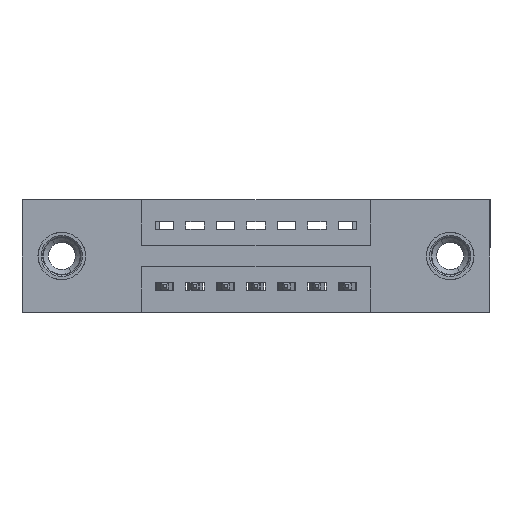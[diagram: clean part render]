
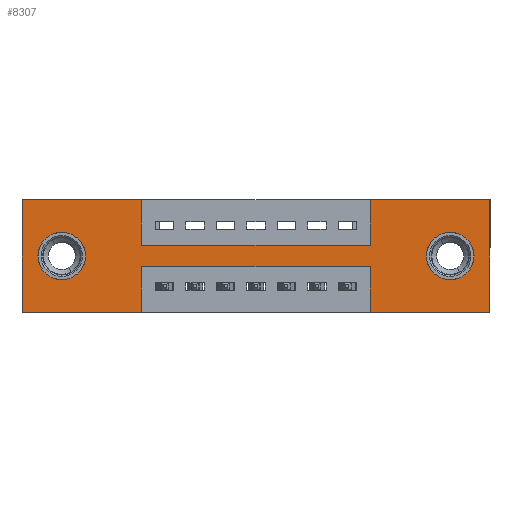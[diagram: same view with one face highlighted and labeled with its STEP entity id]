
A CAD part, front view. The second image highlights one B-rep face of the part: STEP entity #8307.
In plain terms, the highlighted planar face has unit normal (0, -1, 0).
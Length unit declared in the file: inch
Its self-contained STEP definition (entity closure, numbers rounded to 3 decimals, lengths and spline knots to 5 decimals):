
#32 = VERTEX_POINT ( 'NONE', #416 ) ;
#128 = ORIENTED_EDGE ( 'NONE', *, *, #7319, .F. ) ;
#147 = DIRECTION ( 'NONE',  ( 0., 0., -1. ) ) ;
#178 = ORIENTED_EDGE ( 'NONE', *, *, #6725, .F. ) ;
#416 = CARTESIAN_POINT ( 'NONE',  ( 1.1425, 0., -0.37 ) ) ;
#437 = VERTEX_POINT ( 'NONE', #9401 ) ;
#491 = DIRECTION ( 'NONE',  ( 0., -1., 0. ) ) ;
#537 = CARTESIAN_POINT ( 'NONE',  ( 1.535, 0., 0. ) ) ;
#649 = PLANE ( 'NONE',  #10290 ) ;
#993 = CARTESIAN_POINT ( 'NONE',  ( 1.535, 0., 0. ) ) ;
#1049 = EDGE_CURVE ( 'NONE', #6370, #8377, #3163, .T. ) ;
#1101 = DIRECTION ( 'NONE',  ( 0., 0., -1. ) ) ;
#1355 = DIRECTION ( 'NONE',  ( -1., 0., 0. ) ) ;
#1365 = DIRECTION ( 'NONE',  ( 0., 0., -1. ) ) ;
#1394 = CARTESIAN_POINT ( 'NONE',  ( 0.3925, 0., -0.15 ) ) ;
#1626 = CARTESIAN_POINT ( 'NONE',  ( 1.1425, 0., 0. ) ) ;
#1675 = EDGE_CURVE ( 'NONE', #11949, #1896, #2413, .T. ) ;
#1891 = LINE ( 'NONE', #5051, #7633 ) ;
#1896 = VERTEX_POINT ( 'NONE', #8954 ) ;
#1905 = CARTESIAN_POINT ( 'NONE',  ( 0.3925, 0., -0.22 ) ) ;
#1907 = LINE ( 'NONE', #11423, #2347 ) ;
#2055 = VECTOR ( 'NONE', #5692, 39.37008 ) ;
#2180 = VERTEX_POINT ( 'NONE', #1626 ) ;
#2265 = DIRECTION ( 'NONE',  ( 0., 0., 1. ) ) ;
#2316 = CARTESIAN_POINT ( 'NONE',  ( 0.3925, 0., -0.37 ) ) ;
#2347 = VECTOR ( 'NONE', #7662, 39.37008 ) ;
#2413 = LINE ( 'NONE', #993, #10087 ) ;
#2418 = CARTESIAN_POINT ( 'NONE',  ( 0., 0., -0.37 ) ) ;
#2515 = VECTOR ( 'NONE', #6952, 39.37008 ) ;
#2685 = VECTOR ( 'NONE', #8805, 39.37008 ) ;
#2718 = DIRECTION ( 'NONE',  ( 0., 0., 1. ) ) ;
#2781 = LINE ( 'NONE', #10447, #10880 ) ;
#2822 = CARTESIAN_POINT ( 'NONE',  ( 0., 0., 0. ) ) ;
#2894 = DIRECTION ( 'NONE',  ( 0., 0., 1. ) ) ;
#3065 = LINE ( 'NONE', #2418, #10860 ) ;
#3084 = CIRCLE ( 'NONE', #8422, 0.078 ) ;
#3163 = LINE ( 'NONE', #4770, #4205 ) ;
#3208 = CARTESIAN_POINT ( 'NONE',  ( 0.13, 0., -0.107 ) ) ;
#3235 = VERTEX_POINT ( 'NONE', #12100 ) ;
#3254 = VERTEX_POINT ( 'NONE', #10352 ) ;
#3307 = DIRECTION ( 'NONE',  ( 0., 0., -1. ) ) ;
#3404 = LINE ( 'NONE', #11614, #2515 ) ;
#3464 = AXIS2_PLACEMENT_3D ( 'NONE', #3787, #8413, #2718 ) ;
#3496 = ORIENTED_EDGE ( 'NONE', *, *, #7632, .T. ) ;
#3515 = FACE_OUTER_BOUND ( 'NONE', #6228, .T. ) ;
#3522 = ORIENTED_EDGE ( 'NONE', *, *, #11825, .F. ) ;
#3657 = EDGE_CURVE ( 'NONE', #10098, #3861, #11981, .T. ) ;
#3721 = CARTESIAN_POINT ( 'NONE',  ( 0.13, 0., -0.263 ) ) ;
#3787 = CARTESIAN_POINT ( 'NONE',  ( 0.13, 0., -0.185 ) ) ;
#3814 = LINE ( 'NONE', #1905, #9875 ) ;
#3861 = VERTEX_POINT ( 'NONE', #6309 ) ;
#3905 = CARTESIAN_POINT ( 'NONE',  ( 1.405, 0., -0.185 ) ) ;
#4005 = CARTESIAN_POINT ( 'NONE',  ( 0.3925, 0., -0.22 ) ) ;
#4166 = LINE ( 'NONE', #7695, #2685 ) ;
#4205 = VECTOR ( 'NONE', #11273, 39.37008 ) ;
#4251 = VERTEX_POINT ( 'NONE', #11196 ) ;
#4426 = LINE ( 'NONE', #7701, #9264 ) ;
#4716 = VERTEX_POINT ( 'NONE', #2316 ) ;
#4770 = CARTESIAN_POINT ( 'NONE',  ( 0., 0., 0. ) ) ;
#5006 = ORIENTED_EDGE ( 'NONE', *, *, #11823, .F. ) ;
#5051 = CARTESIAN_POINT ( 'NONE',  ( 0., 0., -0.37 ) ) ;
#5293 = DIRECTION ( 'NONE',  ( -1., 0., 0. ) ) ;
#5386 = CARTESIAN_POINT ( 'NONE',  ( 0.3925, 0., 0. ) ) ;
#5692 = DIRECTION ( 'NONE',  ( 0., 0., -1. ) ) ;
#5877 = ORIENTED_EDGE ( 'NONE', *, *, #8700, .F. ) ;
#5997 = DIRECTION ( 'NONE',  ( 0., 0., -1. ) ) ;
#6005 = ORIENTED_EDGE ( 'NONE', *, *, #8075, .F. ) ;
#6096 = EDGE_CURVE ( 'NONE', #8530, #8887, #8306, .T. ) ;
#6140 = VERTEX_POINT ( 'NONE', #4005 ) ;
#6228 = EDGE_LOOP ( 'NONE', ( #5006, #8393, #128, #11039, #8133, #3522, #6005, #6629, #9432, #12099, #178, #5877 ) ) ;
#6309 = CARTESIAN_POINT ( 'NONE',  ( 1.1425, 0., -0.15 ) ) ;
#6370 = VERTEX_POINT ( 'NONE', #2822 ) ;
#6389 = EDGE_LOOP ( 'NONE', ( #11942, #7122 ) ) ;
#6629 = ORIENTED_EDGE ( 'NONE', *, *, #3657, .F. ) ;
#6674 = CIRCLE ( 'NONE', #8797, 0.078 ) ;
#6725 = EDGE_CURVE ( 'NONE', #3235, #6370, #4166, .T. ) ;
#6773 = CIRCLE ( 'NONE', #9696, 0.078 ) ;
#6938 = CARTESIAN_POINT ( 'NONE',  ( 1.405, 0., -0.185 ) ) ;
#6952 = DIRECTION ( 'NONE',  ( 0., 0., 1. ) ) ;
#7122 = ORIENTED_EDGE ( 'NONE', *, *, #6096, .T. ) ;
#7204 = FACE_BOUND ( 'NONE', #11450, .T. ) ;
#7319 = EDGE_CURVE ( 'NONE', #32, #437, #3404, .T. ) ;
#7632 = EDGE_CURVE ( 'NONE', #3254, #4251, #6773, .T. ) ;
#7633 = VECTOR ( 'NONE', #1355, 39.37008 ) ;
#7662 = DIRECTION ( 'NONE',  ( 1., 0., 0. ) ) ;
#7695 = CARTESIAN_POINT ( 'NONE',  ( 0., 0., 0. ) ) ;
#7701 = CARTESIAN_POINT ( 'NONE',  ( 0.3925, 0., -0.37 ) ) ;
#7907 = DIRECTION ( 'NONE',  ( 0., 1., 0. ) ) ;
#7916 = CARTESIAN_POINT ( 'NONE',  ( 0.3925, 0., -0.15 ) ) ;
#8075 = EDGE_CURVE ( 'NONE', #3861, #2180, #2781, .T. ) ;
#8085 = EDGE_CURVE ( 'NONE', #8377, #10098, #8118, .T. ) ;
#8118 = LINE ( 'NONE', #5386, #2055 ) ;
#8133 = ORIENTED_EDGE ( 'NONE', *, *, #1675, .F. ) ;
#8162 = EDGE_CURVE ( 'NONE', #8887, #8530, #3084, .T. ) ;
#8306 = CIRCLE ( 'NONE', #3464, 0.078 ) ;
#8307 = ADVANCED_FACE ( 'NONE', ( #7204, #11883, #3515 ), #649, .T. ) ;
#8377 = VERTEX_POINT ( 'NONE', #11608 ) ;
#8393 = ORIENTED_EDGE ( 'NONE', *, *, #11790, .F. ) ;
#8413 = DIRECTION ( 'NONE',  ( 0., 1., 0. ) ) ;
#8422 = AXIS2_PLACEMENT_3D ( 'NONE', #10681, #7907, #2265 ) ;
#8504 = DIRECTION ( 'NONE',  ( -1., 0., 0. ) ) ;
#8530 = VERTEX_POINT ( 'NONE', #3721 ) ;
#8700 = EDGE_CURVE ( 'NONE', #4716, #3235, #1891, .T. ) ;
#8797 = AXIS2_PLACEMENT_3D ( 'NONE', #3905, #9573, #1101 ) ;
#8805 = DIRECTION ( 'NONE',  ( 0., 0., 1. ) ) ;
#8887 = VERTEX_POINT ( 'NONE', #3208 ) ;
#8954 = CARTESIAN_POINT ( 'NONE',  ( 1.535, 0., -0.37 ) ) ;
#8963 = EDGE_CURVE ( 'NONE', #1896, #32, #3065, .T. ) ;
#9264 = VECTOR ( 'NONE', #5997, 39.37008 ) ;
#9330 = EDGE_CURVE ( 'NONE', #4251, #3254, #6674, .T. ) ;
#9401 = CARTESIAN_POINT ( 'NONE',  ( 1.1425, 0., -0.22 ) ) ;
#9432 = ORIENTED_EDGE ( 'NONE', *, *, #8085, .F. ) ;
#9536 = VECTOR ( 'NONE', #10773, 39.37008 ) ;
#9573 = DIRECTION ( 'NONE',  ( 0., 1., 0. ) ) ;
#9696 = AXIS2_PLACEMENT_3D ( 'NONE', #6938, #10710, #1365 ) ;
#9875 = VECTOR ( 'NONE', #8504, 39.37008 ) ;
#10045 = CARTESIAN_POINT ( 'NONE',  ( 0., 0., -0.37 ) ) ;
#10087 = VECTOR ( 'NONE', #147, 39.37008 ) ;
#10098 = VERTEX_POINT ( 'NONE', #1394 ) ;
#10290 = AXIS2_PLACEMENT_3D ( 'NONE', #10045, #491, #3307 ) ;
#10352 = CARTESIAN_POINT ( 'NONE',  ( 1.405, 0., -0.107 ) ) ;
#10447 = CARTESIAN_POINT ( 'NONE',  ( 1.1425, 0., 0. ) ) ;
#10681 = CARTESIAN_POINT ( 'NONE',  ( 0.13, 0., -0.185 ) ) ;
#10710 = DIRECTION ( 'NONE',  ( 0., 1., 0. ) ) ;
#10773 = DIRECTION ( 'NONE',  ( 1., 0., 0. ) ) ;
#10860 = VECTOR ( 'NONE', #5293, 39.37008 ) ;
#10880 = VECTOR ( 'NONE', #2894, 39.37008 ) ;
#11039 = ORIENTED_EDGE ( 'NONE', *, *, #8963, .F. ) ;
#11196 = CARTESIAN_POINT ( 'NONE',  ( 1.405, 0., -0.263 ) ) ;
#11273 = DIRECTION ( 'NONE',  ( 1., 0., 0. ) ) ;
#11423 = CARTESIAN_POINT ( 'NONE',  ( 0., 0., 0. ) ) ;
#11450 = EDGE_LOOP ( 'NONE', ( #3496, #12165 ) ) ;
#11608 = CARTESIAN_POINT ( 'NONE',  ( 0.3925, 0., 0. ) ) ;
#11614 = CARTESIAN_POINT ( 'NONE',  ( 1.1425, 0., -0.37 ) ) ;
#11790 = EDGE_CURVE ( 'NONE', #437, #6140, #3814, .T. ) ;
#11823 = EDGE_CURVE ( 'NONE', #6140, #4716, #4426, .T. ) ;
#11825 = EDGE_CURVE ( 'NONE', #2180, #11949, #1907, .T. ) ;
#11883 = FACE_BOUND ( 'NONE', #6389, .T. ) ;
#11942 = ORIENTED_EDGE ( 'NONE', *, *, #8162, .T. ) ;
#11949 = VERTEX_POINT ( 'NONE', #537 ) ;
#11981 = LINE ( 'NONE', #7916, #9536 ) ;
#12099 = ORIENTED_EDGE ( 'NONE', *, *, #1049, .F. ) ;
#12100 = CARTESIAN_POINT ( 'NONE',  ( 0., 0., -0.37 ) ) ;
#12165 = ORIENTED_EDGE ( 'NONE', *, *, #9330, .T. ) ;
